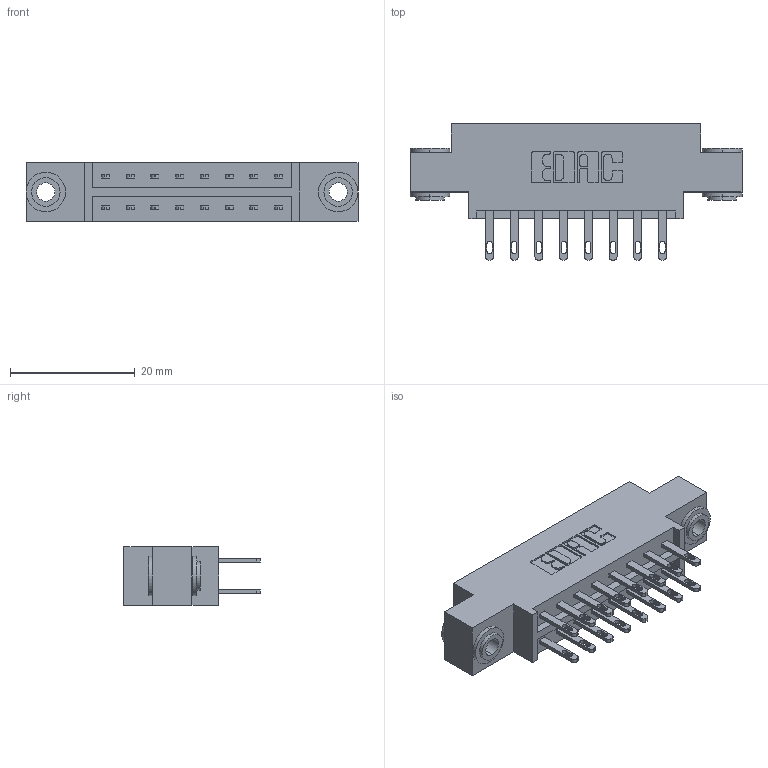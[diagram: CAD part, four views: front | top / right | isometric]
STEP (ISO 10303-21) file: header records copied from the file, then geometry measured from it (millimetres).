
FILE_DESCRIPTION (( 'STEP AP203' ), '1' );
FILE_NAME ('833-016-500-803.STEP', '2020-05-31T16:44:26', ( '' ), ( '' ), 'SwSTEP 2.0', 'SolidWorks 2020', '' );
FILE_SCHEMA (( 'CONFIG_CONTROL_DESIGN' ));
Length unit declared in the file: inch
Products named in the file (4): 833 Part_Offset - .156 Dia - TH; 833-016-500-803; 345-292-001_345-293-100; 345-250-002_345-250-002-102
Assembly tree (19 placements, depth 2):
  833-016-500-803
    833 Part_Offset - .156 Dia - TH
    345-292-001_345-293-100  x16
    345-250-002_345-250-002-102  x2
Bounding box: 53.24 x 21.85 x 9.4 mm (x, y, z)
Volume: 4957.9 mm3; surface area: 6113.9 mm2
Topology: 19 solids, 19 shells, 924 faces, 2751 edges, 1830 vertices
Faces by surface type: plane 564, cylinder 352, cone 8
Entity records: 10256 total; most frequent: CARTESIAN_POINT 1717, ORIENTED_EDGE 1646, DIRECTION 1561, EDGE_CURVE 823, LINE 667, VECTOR 667, VERTEX_POINT 546, AXIS2_PLACEMENT_3D 447
